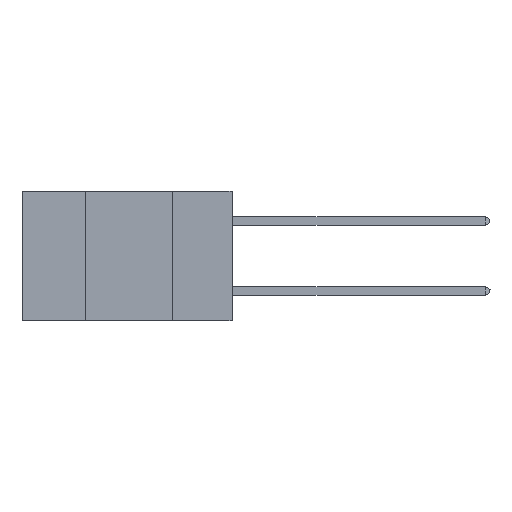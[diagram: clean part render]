
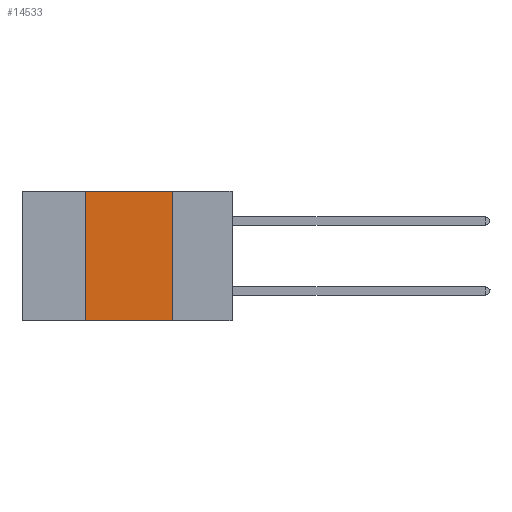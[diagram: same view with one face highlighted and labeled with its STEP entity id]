
A CAD part, left-side view. The second image highlights one B-rep face of the part: STEP entity #14533.
In plain terms, the highlighted planar face has unit normal (-1, 0, 0).
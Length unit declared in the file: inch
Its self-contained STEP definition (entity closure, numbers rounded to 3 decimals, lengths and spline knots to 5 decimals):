
#255 = ORIENTED_EDGE ( 'NONE', *, *, #676, .F. ) ;
#676 = EDGE_CURVE ( 'NONE', #3310, #10744, #18173, .T. ) ;
#841 = CARTESIAN_POINT ( 'NONE',  ( 0., 0.6, -0.37 ) ) ;
#1414 = CARTESIAN_POINT ( 'NONE',  ( 0., 0.17, -0.37 ) ) ;
#2209 = FACE_OUTER_BOUND ( 'NONE', #13249, .T. ) ;
#2433 = VERTEX_POINT ( 'NONE', #9297 ) ;
#3310 = VERTEX_POINT ( 'NONE', #16588 ) ;
#3844 = CARTESIAN_POINT ( 'NONE',  ( 0., 0.6, 0. ) ) ;
#3944 = DIRECTION ( 'NONE',  ( 0., 0., -1. ) ) ;
#5255 = LINE ( 'NONE', #3844, #11038 ) ;
#5339 = DIRECTION ( 'NONE',  ( 0., -1., 0. ) ) ;
#5948 = AXIS2_PLACEMENT_3D ( 'NONE', #7938, #18029, #13541 ) ;
#6184 = VECTOR ( 'NONE', #3944, 39.37008 ) ;
#6237 = ORIENTED_EDGE ( 'NONE', *, *, #12350, .F. ) ;
#7938 = CARTESIAN_POINT ( 'NONE',  ( 0., 0.6, 0. ) ) ;
#8078 = CARTESIAN_POINT ( 'NONE',  ( 0., 0.17, 0. ) ) ;
#8303 = CARTESIAN_POINT ( 'NONE',  ( 0., 0.42, -0.37 ) ) ;
#8986 = ORIENTED_EDGE ( 'NONE', *, *, #10930, .F. ) ;
#9297 = CARTESIAN_POINT ( 'NONE',  ( 0., 0.42, 0. ) ) ;
#10039 = VERTEX_POINT ( 'NONE', #8303 ) ;
#10744 = VERTEX_POINT ( 'NONE', #1414 ) ;
#10930 = EDGE_CURVE ( 'NONE', #2433, #3310, #5255, .T. ) ;
#11022 = DIRECTION ( 'NONE',  ( 0., -1., 0. ) ) ;
#11038 = VECTOR ( 'NONE', #11022, 39.37008 ) ;
#12342 = CARTESIAN_POINT ( 'NONE',  ( 0., 0.42, 0. ) ) ;
#12350 = EDGE_CURVE ( 'NONE', #10039, #2433, #13761, .T. ) ;
#12354 = EDGE_CURVE ( 'NONE', #10039, #10744, #18251, .T. ) ;
#13249 = EDGE_LOOP ( 'NONE', ( #255, #8986, #6237, #14733 ) ) ;
#13456 = VECTOR ( 'NONE', #5339, 39.37008 ) ;
#13541 = DIRECTION ( 'NONE',  ( 0., 0., -1. ) ) ;
#13761 = LINE ( 'NONE', #12342, #17341 ) ;
#14533 = ADVANCED_FACE ( 'NONE', ( #2209 ), #15390, .F. ) ;
#14733 = ORIENTED_EDGE ( 'NONE', *, *, #12354, .T. ) ;
#15390 = PLANE ( 'NONE',  #5948 ) ;
#16588 = CARTESIAN_POINT ( 'NONE',  ( 0., 0.17, 0. ) ) ;
#17341 = VECTOR ( 'NONE', #18065, 39.37008 ) ;
#18029 = DIRECTION ( 'NONE',  ( 1., 0., 0. ) ) ;
#18065 = DIRECTION ( 'NONE',  ( 0., 0., 1. ) ) ;
#18173 = LINE ( 'NONE', #8078, #6184 ) ;
#18251 = LINE ( 'NONE', #841, #13456 ) ;
